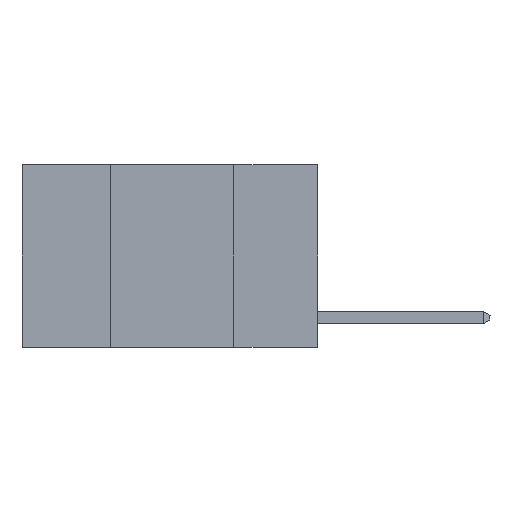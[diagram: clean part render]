
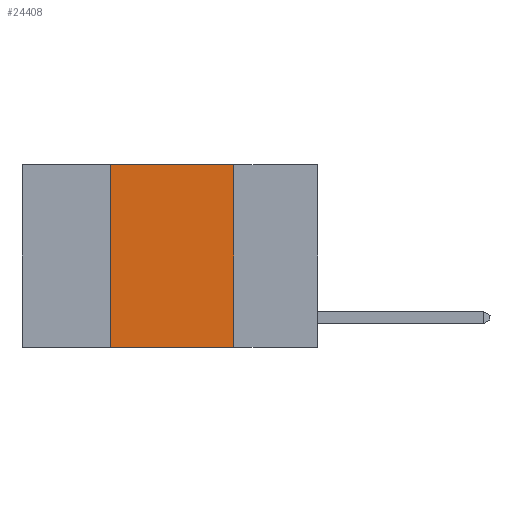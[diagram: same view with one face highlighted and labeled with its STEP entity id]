
A CAD part, left-side view. The second image highlights one B-rep face of the part: STEP entity #24408.
In plain terms, the highlighted planar face has unit normal (-1, 0, 0).
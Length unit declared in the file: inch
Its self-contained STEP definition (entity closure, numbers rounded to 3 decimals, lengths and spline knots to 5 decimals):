
#74 = ORIENTED_EDGE ( 'NONE', *, *, #4726, .F. ) ;
#399 = EDGE_CURVE ( 'NONE', #20316, #1621, #9294, .T. ) ;
#1621 = VERTEX_POINT ( 'NONE', #17052 ) ;
#1785 = DIRECTION ( 'NONE',  ( 0., 0., -1. ) ) ;
#2579 = LINE ( 'NONE', #19135, #17865 ) ;
#3894 = EDGE_CURVE ( 'NONE', #17106, #8024, #16023, .T. ) ;
#4178 = VECTOR ( 'NONE', #22765, 39.37008 ) ;
#4726 = EDGE_CURVE ( 'NONE', #17106, #20316, #2579, .T. ) ;
#4736 = AXIS2_PLACEMENT_3D ( 'NONE', #19769, #23536, #12187 ) ;
#6989 = CARTESIAN_POINT ( 'NONE',  ( 0., 0.17, -0.37 ) ) ;
#8024 = VERTEX_POINT ( 'NONE', #6989 ) ;
#9294 = LINE ( 'NONE', #15143, #4178 ) ;
#10384 = ORIENTED_EDGE ( 'NONE', *, *, #3894, .T. ) ;
#10953 = VECTOR ( 'NONE', #24401, 39.37008 ) ;
#11092 = CARTESIAN_POINT ( 'NONE',  ( 0., 0.6, -0.37 ) ) ;
#11156 = EDGE_CURVE ( 'NONE', #1621, #8024, #21853, .T. ) ;
#11171 = VECTOR ( 'NONE', #1785, 39.37008 ) ;
#12187 = DIRECTION ( 'NONE',  ( 0., 0., -1. ) ) ;
#12467 = DIRECTION ( 'NONE',  ( 0., 0., 1. ) ) ;
#12867 = FACE_OUTER_BOUND ( 'NONE', #21755, .T. ) ;
#14809 = ORIENTED_EDGE ( 'NONE', *, *, #399, .F. ) ;
#15143 = CARTESIAN_POINT ( 'NONE',  ( 0., 0.6, 0. ) ) ;
#15188 = CARTESIAN_POINT ( 'NONE',  ( 0., 0.17, 0. ) ) ;
#15941 = PLANE ( 'NONE',  #4736 ) ;
#16023 = LINE ( 'NONE', #11092, #10953 ) ;
#17052 = CARTESIAN_POINT ( 'NONE',  ( 0., 0.17, 0. ) ) ;
#17106 = VERTEX_POINT ( 'NONE', #21314 ) ;
#17865 = VECTOR ( 'NONE', #12467, 39.37008 ) ;
#19135 = CARTESIAN_POINT ( 'NONE',  ( 0., 0.42, 0. ) ) ;
#19295 = ORIENTED_EDGE ( 'NONE', *, *, #11156, .F. ) ;
#19769 = CARTESIAN_POINT ( 'NONE',  ( 0., 0.6, 0. ) ) ;
#20041 = CARTESIAN_POINT ( 'NONE',  ( 0., 0.42, 0. ) ) ;
#20316 = VERTEX_POINT ( 'NONE', #20041 ) ;
#21314 = CARTESIAN_POINT ( 'NONE',  ( 0., 0.42, -0.37 ) ) ;
#21755 = EDGE_LOOP ( 'NONE', ( #19295, #14809, #74, #10384 ) ) ;
#21853 = LINE ( 'NONE', #15188, #11171 ) ;
#22765 = DIRECTION ( 'NONE',  ( 0., -1., 0. ) ) ;
#23536 = DIRECTION ( 'NONE',  ( 1., 0., 0. ) ) ;
#24401 = DIRECTION ( 'NONE',  ( 0., -1., 0. ) ) ;
#24408 = ADVANCED_FACE ( 'NONE', ( #12867 ), #15941, .F. ) ;
